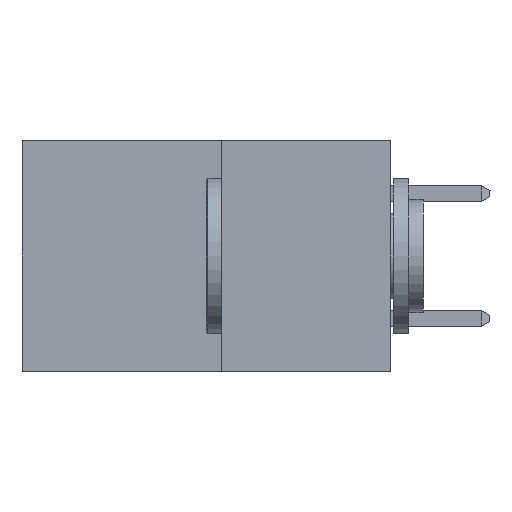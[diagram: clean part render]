
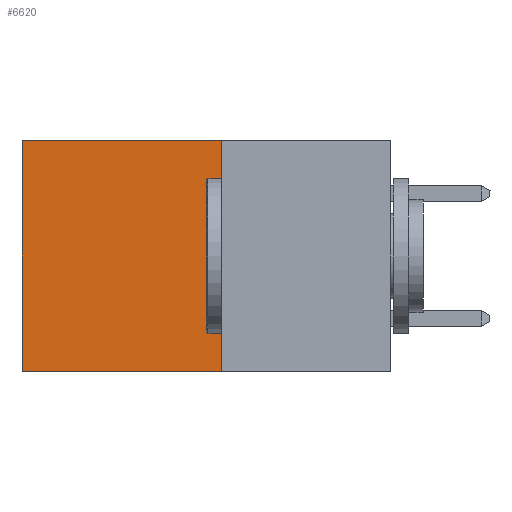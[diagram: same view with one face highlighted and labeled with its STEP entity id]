
A CAD part, left-side view. The second image highlights one B-rep face of the part: STEP entity #6620.
In plain terms, the highlighted planar face has unit normal (-1, 0, 0).
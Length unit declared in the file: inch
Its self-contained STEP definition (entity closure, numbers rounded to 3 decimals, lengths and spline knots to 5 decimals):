
#1495 = CARTESIAN_POINT ( 'NONE',  ( 0.277, 0.59, -0.37 ) ) ;
#2234 = ORIENTED_EDGE ( 'NONE', *, *, #3504, .T. ) ;
#2403 = LINE ( 'NONE', #12852, #8747 ) ;
#3458 = DIRECTION ( 'NONE',  ( 0., 0., -1. ) ) ;
#3504 = EDGE_CURVE ( 'NONE', #11946, #9013, #2403, .T. ) ;
#5246 = LINE ( 'NONE', #10585, #9205 ) ;
#5399 = AXIS2_PLACEMENT_3D ( 'NONE', #11957, #11888, #11861 ) ;
#5468 = VERTEX_POINT ( 'NONE', #8707 ) ;
#6139 = CARTESIAN_POINT ( 'NONE',  ( 0.277, 0.59, 0. ) ) ;
#6519 = CARTESIAN_POINT ( 'NONE',  ( 0.277, 0.27, -0.37 ) ) ;
#6620 = ADVANCED_FACE ( 'NONE', ( #10139 ), #11929, .F. ) ;
#6981 = DIRECTION ( 'NONE',  ( 0., 1., 0. ) ) ;
#8490 = LINE ( 'NONE', #12845, #14238 ) ;
#8682 = VECTOR ( 'NONE', #8902, 39.37008 ) ;
#8707 = CARTESIAN_POINT ( 'NONE',  ( 0.277, 0.27, -0.37 ) ) ;
#8747 = VECTOR ( 'NONE', #12773, 39.37008 ) ;
#8777 = EDGE_CURVE ( 'NONE', #9013, #11876, #5246, .T. ) ;
#8902 = DIRECTION ( 'NONE',  ( 0., 0., -1. ) ) ;
#9013 = VERTEX_POINT ( 'NONE', #6139 ) ;
#9066 = LINE ( 'NONE', #6519, #8682 ) ;
#9205 = VECTOR ( 'NONE', #3458, 39.37008 ) ;
#10139 = FACE_OUTER_BOUND ( 'NONE', #13495, .T. ) ;
#10585 = CARTESIAN_POINT ( 'NONE',  ( 0.277, 0.59, -0.37 ) ) ;
#10742 = ORIENTED_EDGE ( 'NONE', *, *, #13620, .F. ) ;
#11861 = DIRECTION ( 'NONE',  ( 0., 0., -1. ) ) ;
#11876 = VERTEX_POINT ( 'NONE', #1495 ) ;
#11888 = DIRECTION ( 'NONE',  ( 1., 0., 0. ) ) ;
#11929 = PLANE ( 'NONE',  #5399 ) ;
#11946 = VERTEX_POINT ( 'NONE', #12293 ) ;
#11957 = CARTESIAN_POINT ( 'NONE',  ( 0.277, 0.27, -0.37 ) ) ;
#12231 = ORIENTED_EDGE ( 'NONE', *, *, #13381, .F. ) ;
#12293 = CARTESIAN_POINT ( 'NONE',  ( 0.277, 0.27, 0. ) ) ;
#12465 = ORIENTED_EDGE ( 'NONE', *, *, #8777, .T. ) ;
#12773 = DIRECTION ( 'NONE',  ( 0., 1., 0. ) ) ;
#12845 = CARTESIAN_POINT ( 'NONE',  ( 0.277, 0.27, -0.37 ) ) ;
#12852 = CARTESIAN_POINT ( 'NONE',  ( 0.277, 0.27, 0. ) ) ;
#13381 = EDGE_CURVE ( 'NONE', #11946, #5468, #9066, .T. ) ;
#13495 = EDGE_LOOP ( 'NONE', ( #12465, #10742, #12231, #2234 ) ) ;
#13620 = EDGE_CURVE ( 'NONE', #5468, #11876, #8490, .T. ) ;
#14238 = VECTOR ( 'NONE', #6981, 39.37008 ) ;
